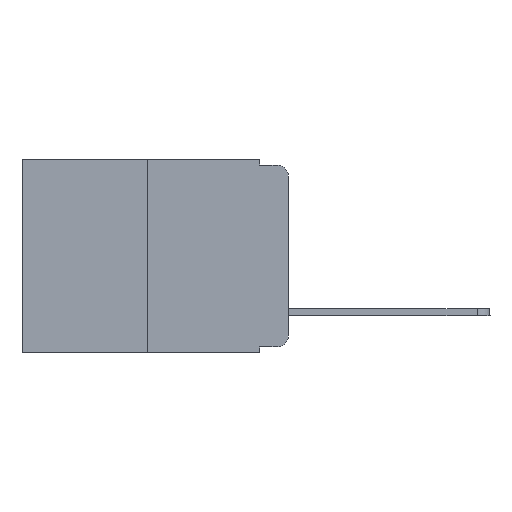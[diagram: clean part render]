
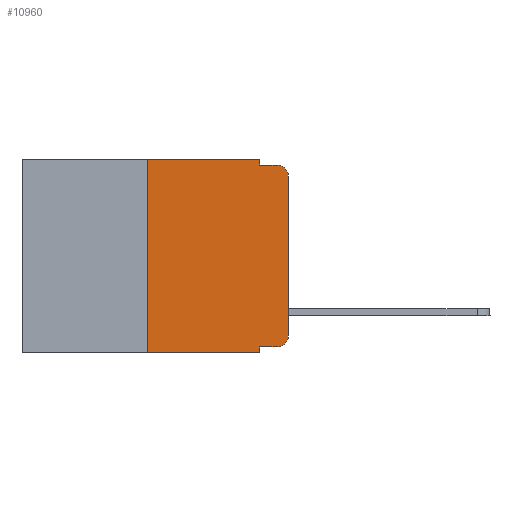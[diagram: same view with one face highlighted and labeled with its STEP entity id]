
A CAD part, left-side view. The second image highlights one B-rep face of the part: STEP entity #10960.
In plain terms, the highlighted planar face has unit normal (-1, 0, 0).
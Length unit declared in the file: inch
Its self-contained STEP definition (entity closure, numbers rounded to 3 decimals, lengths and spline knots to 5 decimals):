
#596 = ORIENTED_EDGE ( 'NONE', *, *, #12804, .F. ) ;
#758 = DIRECTION ( 'NONE',  ( 0., 0., 1. ) ) ;
#769 = LINE ( 'NONE', #787, #1238 ) ;
#787 = CARTESIAN_POINT ( 'NONE',  ( 0., 0.051, -0.01 ) ) ;
#837 = VERTEX_POINT ( 'NONE', #5781 ) ;
#950 = CARTESIAN_POINT ( 'NONE',  ( 0., 0., 0. ) ) ;
#1028 = AXIS2_PLACEMENT_3D ( 'NONE', #12931, #11218, #15941 ) ;
#1075 = VERTEX_POINT ( 'NONE', #1810 ) ;
#1238 = VECTOR ( 'NONE', #14872, 39.37008 ) ;
#1659 = EDGE_CURVE ( 'NONE', #1898, #19027, #3575, .T. ) ;
#1766 = DIRECTION ( 'NONE',  ( 0., -1., 0. ) ) ;
#1797 = PLANE ( 'NONE',  #10219 ) ;
#1810 = CARTESIAN_POINT ( 'NONE',  ( 0., 0.051, 0. ) ) ;
#1898 = VERTEX_POINT ( 'NONE', #17782 ) ;
#2156 = EDGE_CURVE ( 'NONE', #1075, #3939, #20190, .T. ) ;
#2371 = CARTESIAN_POINT ( 'NONE',  ( 0., 0.02, -0.333 ) ) ;
#2527 = ORIENTED_EDGE ( 'NONE', *, *, #17992, .T. ) ;
#2707 = VERTEX_POINT ( 'NONE', #14668 ) ;
#3575 = LINE ( 'NONE', #14194, #19234 ) ;
#3939 = VERTEX_POINT ( 'NONE', #11613 ) ;
#4288 = DIRECTION ( 'NONE',  ( 0., 0., 1. ) ) ;
#4307 = VECTOR ( 'NONE', #15716, 39.37008 ) ;
#4740 = DIRECTION ( 'NONE',  ( 0., 0., -1. ) ) ;
#5028 = EDGE_CURVE ( 'NONE', #12965, #1075, #9655, .T. ) ;
#5388 = VECTOR ( 'NONE', #13866, 39.37008 ) ;
#5781 = CARTESIAN_POINT ( 'NONE',  ( 0., 0.25, -0.343 ) ) ;
#5921 = VERTEX_POINT ( 'NONE', #18242 ) ;
#5994 = VECTOR ( 'NONE', #11700, 39.37008 ) ;
#6249 = FACE_OUTER_BOUND ( 'NONE', #16377, .T. ) ;
#6474 = ORIENTED_EDGE ( 'NONE', *, *, #14370, .T. ) ;
#7258 = LINE ( 'NONE', #15155, #8451 ) ;
#7615 = AXIS2_PLACEMENT_3D ( 'NONE', #17114, #14229, #4740 ) ;
#7980 = DIRECTION ( 'NONE',  ( 1., 0., 0. ) ) ;
#8045 = VECTOR ( 'NONE', #758, 39.37008 ) ;
#8357 = VERTEX_POINT ( 'NONE', #14764 ) ;
#8451 = VECTOR ( 'NONE', #4288, 39.37008 ) ;
#8704 = EDGE_CURVE ( 'NONE', #1898, #8357, #16889, .T. ) ;
#9124 = VERTEX_POINT ( 'NONE', #16431 ) ;
#9316 = CARTESIAN_POINT ( 'NONE',  ( 0., 0.25, 0. ) ) ;
#9655 = LINE ( 'NONE', #18791, #4307 ) ;
#9987 = ORIENTED_EDGE ( 'NONE', *, *, #1659, .T. ) ;
#10219 = AXIS2_PLACEMENT_3D ( 'NONE', #16926, #7980, #18504 ) ;
#10960 = ADVANCED_FACE ( 'NONE', ( #6249 ), #1797, .F. ) ;
#11011 = ORIENTED_EDGE ( 'NONE', *, *, #17716, .F. ) ;
#11121 = DIRECTION ( 'NONE',  ( 0., -1., 0. ) ) ;
#11218 = DIRECTION ( 'NONE',  ( -1., 0., 0. ) ) ;
#11613 = CARTESIAN_POINT ( 'NONE',  ( 0., 0.051, -0.01 ) ) ;
#11700 = DIRECTION ( 'NONE',  ( 0., 0., -1. ) ) ;
#11855 = EDGE_CURVE ( 'NONE', #9124, #5921, #19434, .T. ) ;
#11880 = CIRCLE ( 'NONE', #1028, 0.02 ) ;
#12356 = LINE ( 'NONE', #14434, #15072 ) ;
#12579 = ORIENTED_EDGE ( 'NONE', *, *, #8704, .F. ) ;
#12804 = EDGE_CURVE ( 'NONE', #3939, #5921, #769, .T. ) ;
#12931 = CARTESIAN_POINT ( 'NONE',  ( 0., 0.02, -0.313 ) ) ;
#12965 = VERTEX_POINT ( 'NONE', #9316 ) ;
#13753 = ORIENTED_EDGE ( 'NONE', *, *, #5028, .F. ) ;
#13805 = CARTESIAN_POINT ( 'NONE',  ( 0., 0.051, 0. ) ) ;
#13866 = DIRECTION ( 'NONE',  ( 0., 0., -1. ) ) ;
#14130 = ORIENTED_EDGE ( 'NONE', *, *, #11855, .T. ) ;
#14194 = CARTESIAN_POINT ( 'NONE',  ( 0., 0.051, -0.333 ) ) ;
#14229 = DIRECTION ( 'NONE',  ( -1., 0., 0. ) ) ;
#14370 = EDGE_CURVE ( 'NONE', #2707, #9124, #16375, .T. ) ;
#14434 = CARTESIAN_POINT ( 'NONE',  ( 0., 0.473, -0.343 ) ) ;
#14668 = CARTESIAN_POINT ( 'NONE',  ( 0., 0., -0.313 ) ) ;
#14764 = CARTESIAN_POINT ( 'NONE',  ( 0., 0.051, -0.343 ) ) ;
#14872 = DIRECTION ( 'NONE',  ( 0., -1., 0. ) ) ;
#15072 = VECTOR ( 'NONE', #1766, 39.37008 ) ;
#15155 = CARTESIAN_POINT ( 'NONE',  ( 0., 0.25, 0. ) ) ;
#15711 = ORIENTED_EDGE ( 'NONE', *, *, #17896, .T. ) ;
#15716 = DIRECTION ( 'NONE',  ( 0., -1., 0. ) ) ;
#15941 = DIRECTION ( 'NONE',  ( 0., 0., -1. ) ) ;
#16375 = LINE ( 'NONE', #950, #8045 ) ;
#16377 = EDGE_LOOP ( 'NONE', ( #6474, #14130, #596, #17507, #13753, #11011, #15711, #12579, #9987, #2527 ) ) ;
#16431 = CARTESIAN_POINT ( 'NONE',  ( 0., 0., -0.03 ) ) ;
#16889 = LINE ( 'NONE', #13805, #5388 ) ;
#16926 = CARTESIAN_POINT ( 'NONE',  ( 0., 0.473, 0. ) ) ;
#17114 = CARTESIAN_POINT ( 'NONE',  ( 0., 0.02, -0.03 ) ) ;
#17507 = ORIENTED_EDGE ( 'NONE', *, *, #2156, .F. ) ;
#17716 = EDGE_CURVE ( 'NONE', #837, #12965, #7258, .T. ) ;
#17782 = CARTESIAN_POINT ( 'NONE',  ( 0., 0.051, -0.333 ) ) ;
#17896 = EDGE_CURVE ( 'NONE', #837, #8357, #12356, .T. ) ;
#17992 = EDGE_CURVE ( 'NONE', #19027, #2707, #11880, .T. ) ;
#18242 = CARTESIAN_POINT ( 'NONE',  ( 0., 0.02, -0.01 ) ) ;
#18504 = DIRECTION ( 'NONE',  ( 0., 0., -1. ) ) ;
#18791 = CARTESIAN_POINT ( 'NONE',  ( 0., 0.473, 0. ) ) ;
#19027 = VERTEX_POINT ( 'NONE', #2371 ) ;
#19234 = VECTOR ( 'NONE', #11121, 39.37008 ) ;
#19434 = CIRCLE ( 'NONE', #7615, 0.02 ) ;
#19623 = CARTESIAN_POINT ( 'NONE',  ( 0., 0.051, 0. ) ) ;
#20190 = LINE ( 'NONE', #19623, #5994 ) ;
